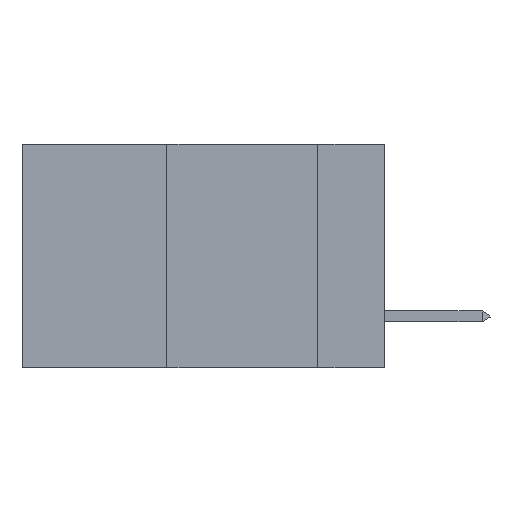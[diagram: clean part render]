
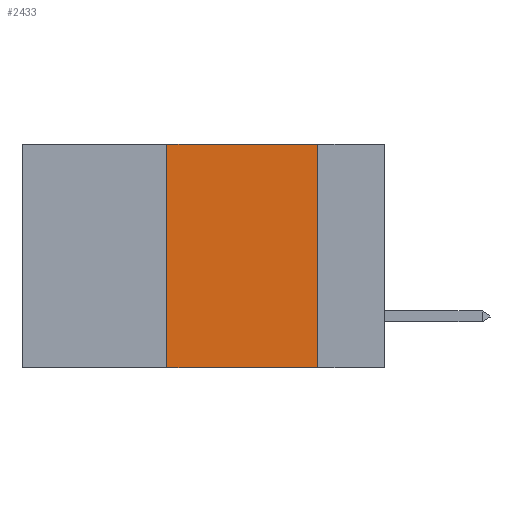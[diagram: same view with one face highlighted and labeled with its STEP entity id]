
A CAD part, left-side view. The second image highlights one B-rep face of the part: STEP entity #2433.
In plain terms, the highlighted planar face has unit normal (-1, 0, 0).
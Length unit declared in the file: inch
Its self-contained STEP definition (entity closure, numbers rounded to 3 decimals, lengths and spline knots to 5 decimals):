
#807 = CARTESIAN_POINT ( 'NONE',  ( 0., 0.11, 0. ) ) ;
#861 = PLANE ( 'NONE',  #16519 ) ;
#1122 = EDGE_CURVE ( 'NONE', #8355, #5830, #7804, .T. ) ;
#1245 = CARTESIAN_POINT ( 'NONE',  ( 0., 0.6, 0. ) ) ;
#2433 = ADVANCED_FACE ( 'NONE', ( #13552 ), #861, .F. ) ;
#5494 = DIRECTION ( 'NONE',  ( 1., 0., 0. ) ) ;
#5830 = VERTEX_POINT ( 'NONE', #28191 ) ;
#6250 = DIRECTION ( 'NONE',  ( 0., -1., 0. ) ) ;
#6261 = EDGE_LOOP ( 'NONE', ( #13616, #11740, #25006, #11765 ) ) ;
#6940 = CARTESIAN_POINT ( 'NONE',  ( 0., 0.36, 0. ) ) ;
#7804 = LINE ( 'NONE', #1245, #27159 ) ;
#8355 = VERTEX_POINT ( 'NONE', #11294 ) ;
#9366 = DIRECTION ( 'NONE',  ( 0., 0., -1. ) ) ;
#9936 = EDGE_CURVE ( 'NONE', #5830, #26106, #18199, .T. ) ;
#11294 = CARTESIAN_POINT ( 'NONE',  ( 0., 0.36, 0. ) ) ;
#11740 = ORIENTED_EDGE ( 'NONE', *, *, #1122, .F. ) ;
#11765 = ORIENTED_EDGE ( 'NONE', *, *, #21016, .T. ) ;
#13225 = LINE ( 'NONE', #21803, #27395 ) ;
#13552 = FACE_OUTER_BOUND ( 'NONE', #6261, .T. ) ;
#13616 = ORIENTED_EDGE ( 'NONE', *, *, #9936, .F. ) ;
#13778 = LINE ( 'NONE', #6940, #18596 ) ;
#14849 = VERTEX_POINT ( 'NONE', #19809 ) ;
#15483 = VECTOR ( 'NONE', #9366, 39.37008 ) ;
#15837 = DIRECTION ( 'NONE',  ( 0., 0., 1. ) ) ;
#16519 = AXIS2_PLACEMENT_3D ( 'NONE', #20784, #5494, #27678 ) ;
#18199 = LINE ( 'NONE', #807, #15483 ) ;
#18596 = VECTOR ( 'NONE', #15837, 39.37008 ) ;
#19809 = CARTESIAN_POINT ( 'NONE',  ( 0., 0.36, -0.37 ) ) ;
#20784 = CARTESIAN_POINT ( 'NONE',  ( 0., 0.6, 0. ) ) ;
#20786 = DIRECTION ( 'NONE',  ( 0., -1., 0. ) ) ;
#21016 = EDGE_CURVE ( 'NONE', #14849, #26106, #13225, .T. ) ;
#21803 = CARTESIAN_POINT ( 'NONE',  ( 0., 0.6, -0.37 ) ) ;
#24581 = CARTESIAN_POINT ( 'NONE',  ( 0., 0.11, -0.37 ) ) ;
#25006 = ORIENTED_EDGE ( 'NONE', *, *, #26793, .F. ) ;
#26106 = VERTEX_POINT ( 'NONE', #24581 ) ;
#26793 = EDGE_CURVE ( 'NONE', #14849, #8355, #13778, .T. ) ;
#27159 = VECTOR ( 'NONE', #20786, 39.37008 ) ;
#27395 = VECTOR ( 'NONE', #6250, 39.37008 ) ;
#27678 = DIRECTION ( 'NONE',  ( 0., 0., -1. ) ) ;
#28191 = CARTESIAN_POINT ( 'NONE',  ( 0., 0.11, 0. ) ) ;
